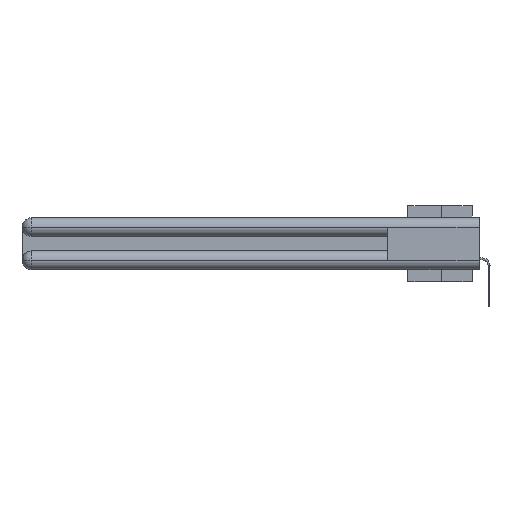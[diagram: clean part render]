
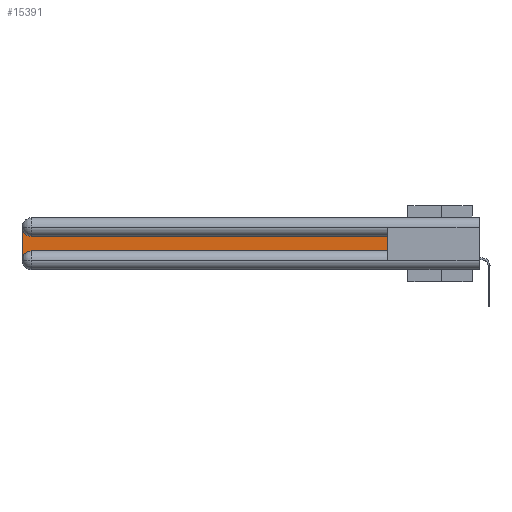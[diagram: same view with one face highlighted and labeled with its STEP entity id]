
A CAD part, left-side view. The second image highlights one B-rep face of the part: STEP entity #15391.
In plain terms, the highlighted planar face has unit normal (-1, 0, 0).
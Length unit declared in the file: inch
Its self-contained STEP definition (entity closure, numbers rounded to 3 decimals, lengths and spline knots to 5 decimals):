
#1258 = DIRECTION ( 'NONE',  ( 1., 0., 0. ) ) ;
#2856 = CARTESIAN_POINT ( 'NONE',  ( 0.075, 2.94, -0.1225 ) ) ;
#3675 = EDGE_LOOP ( 'NONE', ( #26827, #28330, #8842, #26974, #19684, #16144 ) ) ;
#4391 = LINE ( 'NONE', #15000, #22494 ) ;
#4471 = CARTESIAN_POINT ( 'NONE',  ( 0.075, 2.94, -0.2175 ) ) ;
#5130 = EDGE_CURVE ( 'NONE', #18475, #17762, #31515, .T. ) ;
#7250 = CARTESIAN_POINT ( 'NONE',  ( 0.075, 0.6, -0.1225 ) ) ;
#8098 = DIRECTION ( 'NONE',  ( 0., 0., 1. ) ) ;
#8842 = ORIENTED_EDGE ( 'NONE', *, *, #11733, .T. ) ;
#9260 = EDGE_CURVE ( 'NONE', #21869, #10625, #16294, .T. ) ;
#9857 = DIRECTION ( 'NONE',  ( 1., 0., 0. ) ) ;
#9903 = PLANE ( 'NONE',  #11428 ) ;
#10070 = EDGE_CURVE ( 'NONE', #10625, #32228, #25718, .T. ) ;
#10578 = CARTESIAN_POINT ( 'NONE',  ( 0.075, 0.6, -0.2175 ) ) ;
#10625 = VERTEX_POINT ( 'NONE', #31163 ) ;
#11428 = AXIS2_PLACEMENT_3D ( 'NONE', #27861, #30354, #20040 ) ;
#11733 = EDGE_CURVE ( 'NONE', #17762, #13648, #4391, .T. ) ;
#11790 = DIRECTION ( 'NONE',  ( 0., -1., 0. ) ) ;
#12345 = DIRECTION ( 'NONE',  ( 0., 0., -1. ) ) ;
#13648 = VERTEX_POINT ( 'NONE', #29404 ) ;
#14032 = EDGE_CURVE ( 'NONE', #13648, #21869, #24634, .T. ) ;
#14275 = CARTESIAN_POINT ( 'NONE',  ( 0.075, 0.6, -0.2175 ) ) ;
#15000 = CARTESIAN_POINT ( 'NONE',  ( 0.075, 3., -0.2175 ) ) ;
#15254 = DIRECTION ( 'NONE',  ( 0., 1., 0. ) ) ;
#15391 = ADVANCED_FACE ( 'NONE', ( #25029 ), #9903, .F. ) ;
#16144 = ORIENTED_EDGE ( 'NONE', *, *, #10070, .T. ) ;
#16294 = LINE ( 'NONE', #14275, #17878 ) ;
#16519 = CARTESIAN_POINT ( 'NONE',  ( 0.075, 3., -0.0625 ) ) ;
#17070 = EDGE_CURVE ( 'NONE', #32228, #18475, #29737, .T. ) ;
#17492 = CARTESIAN_POINT ( 'NONE',  ( 0.075, 2.94, -0.2775 ) ) ;
#17753 = CARTESIAN_POINT ( 'NONE',  ( 0.075, 0.6, -0.1225 ) ) ;
#17762 = VERTEX_POINT ( 'NONE', #16519 ) ;
#17878 = VECTOR ( 'NONE', #11790, 39.37008 ) ;
#18475 = VERTEX_POINT ( 'NONE', #2856 ) ;
#19281 = AXIS2_PLACEMENT_3D ( 'NONE', #21696, #1258, #26360 ) ;
#19438 = VECTOR ( 'NONE', #8098, 39.37008 ) ;
#19684 = ORIENTED_EDGE ( 'NONE', *, *, #9260, .T. ) ;
#20040 = DIRECTION ( 'NONE',  ( 0., 0., -1. ) ) ;
#20391 = AXIS2_PLACEMENT_3D ( 'NONE', #17492, #9857, #29977 ) ;
#21696 = CARTESIAN_POINT ( 'NONE',  ( 0.075, 2.94, -0.0625 ) ) ;
#21869 = VERTEX_POINT ( 'NONE', #4471 ) ;
#22494 = VECTOR ( 'NONE', #12345, 39.37008 ) ;
#24634 = CIRCLE ( 'NONE', #20391, 0.06 ) ;
#25029 = FACE_OUTER_BOUND ( 'NONE', #3675, .T. ) ;
#25718 = LINE ( 'NONE', #10578, #19438 ) ;
#26360 = DIRECTION ( 'NONE',  ( 0., 0., -1. ) ) ;
#26827 = ORIENTED_EDGE ( 'NONE', *, *, #17070, .T. ) ;
#26974 = ORIENTED_EDGE ( 'NONE', *, *, #14032, .T. ) ;
#27861 = CARTESIAN_POINT ( 'NONE',  ( 0.075, 3., -0.1225 ) ) ;
#28330 = ORIENTED_EDGE ( 'NONE', *, *, #5130, .T. ) ;
#29404 = CARTESIAN_POINT ( 'NONE',  ( 0.075, 3., -0.2775 ) ) ;
#29562 = VECTOR ( 'NONE', #15254, 39.37008 ) ;
#29737 = LINE ( 'NONE', #17753, #29562 ) ;
#29977 = DIRECTION ( 'NONE',  ( 0., 0., -1. ) ) ;
#30354 = DIRECTION ( 'NONE',  ( 1., 0., 0. ) ) ;
#31163 = CARTESIAN_POINT ( 'NONE',  ( 0.075, 0.6, -0.2175 ) ) ;
#31515 = CIRCLE ( 'NONE', #19281, 0.06 ) ;
#32228 = VERTEX_POINT ( 'NONE', #7250 ) ;
